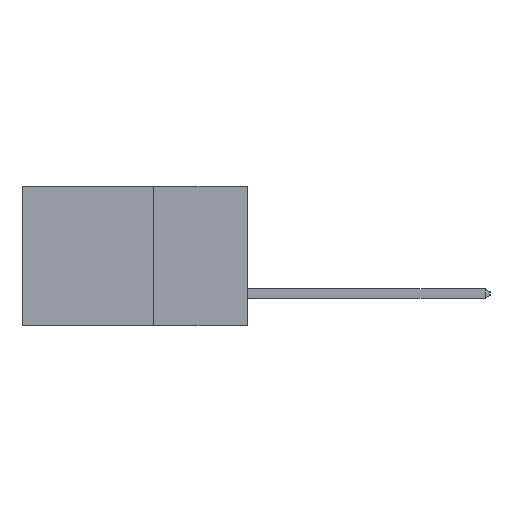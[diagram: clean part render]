
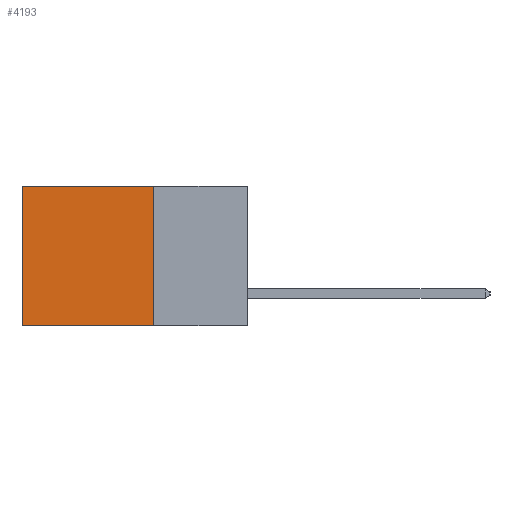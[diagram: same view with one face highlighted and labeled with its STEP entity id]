
A CAD part, left-side view. The second image highlights one B-rep face of the part: STEP entity #4193.
In plain terms, the highlighted planar face has unit normal (-1, 0, 0).
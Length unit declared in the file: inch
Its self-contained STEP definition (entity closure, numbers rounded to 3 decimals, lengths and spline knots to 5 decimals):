
#382 = CARTESIAN_POINT ( 'NONE',  ( 0.298, 0.6, -0.37 ) ) ;
#1085 = CARTESIAN_POINT ( 'NONE',  ( 0.298, 0.25, -0.37 ) ) ;
#1433 = CARTESIAN_POINT ( 'NONE',  ( 0.298, 0.25, -0.37 ) ) ;
#1797 = VECTOR ( 'NONE', #3008, 39.37008 ) ;
#2396 = EDGE_CURVE ( 'NONE', #7282, #15814, #10066, .T. ) ;
#3008 = DIRECTION ( 'NONE',  ( 0., 0., -1. ) ) ;
#3082 = EDGE_CURVE ( 'NONE', #6221, #15814, #5940, .T. ) ;
#4081 = ORIENTED_EDGE ( 'NONE', *, *, #2396, .T. ) ;
#4193 = ADVANCED_FACE ( 'NONE', ( #17124 ), #18916, .F. ) ;
#5810 = LINE ( 'NONE', #17132, #9937 ) ;
#5940 = LINE ( 'NONE', #1433, #6420 ) ;
#6221 = VERTEX_POINT ( 'NONE', #1085 ) ;
#6261 = LINE ( 'NONE', #12043, #18127 ) ;
#6420 = VECTOR ( 'NONE', #15463, 39.37008 ) ;
#7282 = VERTEX_POINT ( 'NONE', #17827 ) ;
#8251 = DIRECTION ( 'NONE',  ( 0., 0., -1. ) ) ;
#9937 = VECTOR ( 'NONE', #8251, 39.37008 ) ;
#10066 = LINE ( 'NONE', #12665, #1797 ) ;
#10434 = ORIENTED_EDGE ( 'NONE', *, *, #15493, .T. ) ;
#11188 = ORIENTED_EDGE ( 'NONE', *, *, #17714, .F. ) ;
#12043 = CARTESIAN_POINT ( 'NONE',  ( 0.298, 0.25, 0. ) ) ;
#12665 = CARTESIAN_POINT ( 'NONE',  ( 0.298, 0.6, 0. ) ) ;
#13647 = CARTESIAN_POINT ( 'NONE',  ( 0.298, 0.25, 0. ) ) ;
#14885 = DIRECTION ( 'NONE',  ( 0., 1., 0. ) ) ;
#15463 = DIRECTION ( 'NONE',  ( 0., 1., 0. ) ) ;
#15493 = EDGE_CURVE ( 'NONE', #17931, #7282, #6261, .T. ) ;
#15814 = VERTEX_POINT ( 'NONE', #382 ) ;
#16146 = EDGE_LOOP ( 'NONE', ( #4081, #16331, #11188, #10434 ) ) ;
#16309 = AXIS2_PLACEMENT_3D ( 'NONE', #19249, #18263, #18240 ) ;
#16331 = ORIENTED_EDGE ( 'NONE', *, *, #3082, .F. ) ;
#17124 = FACE_OUTER_BOUND ( 'NONE', #16146, .T. ) ;
#17132 = CARTESIAN_POINT ( 'NONE',  ( 0.298, 0.25, 0. ) ) ;
#17714 = EDGE_CURVE ( 'NONE', #17931, #6221, #5810, .T. ) ;
#17827 = CARTESIAN_POINT ( 'NONE',  ( 0.298, 0.6, 0. ) ) ;
#17931 = VERTEX_POINT ( 'NONE', #13647 ) ;
#18127 = VECTOR ( 'NONE', #14885, 39.37008 ) ;
#18240 = DIRECTION ( 'NONE',  ( 0., 0., -1. ) ) ;
#18263 = DIRECTION ( 'NONE',  ( 1., 0., 0. ) ) ;
#18916 = PLANE ( 'NONE',  #16309 ) ;
#19249 = CARTESIAN_POINT ( 'NONE',  ( 0.298, 0.25, 0. ) ) ;
